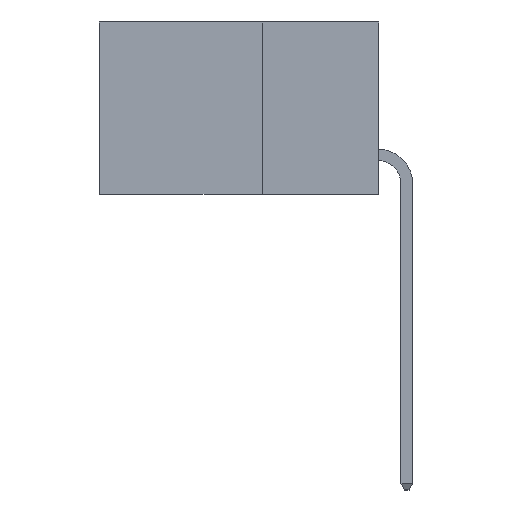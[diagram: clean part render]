
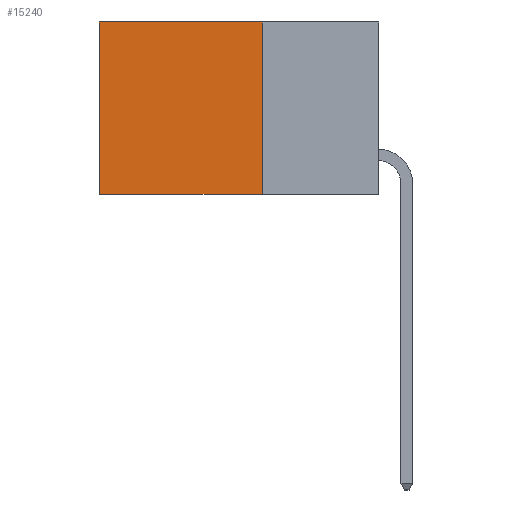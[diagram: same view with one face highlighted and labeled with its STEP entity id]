
A CAD part, left-side view. The second image highlights one B-rep face of the part: STEP entity #15240.
In plain terms, the highlighted planar face has unit normal (-1, 0, 0).
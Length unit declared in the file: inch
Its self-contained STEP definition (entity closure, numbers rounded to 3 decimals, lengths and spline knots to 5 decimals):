
#1170 = CARTESIAN_POINT ( 'NONE',  ( 0.2615, 0.6, -0.37 ) ) ;
#1968 = VERTEX_POINT ( 'NONE', #3800 ) ;
#2512 = LINE ( 'NONE', #5197, #6730 ) ;
#2752 = PLANE ( 'NONE',  #13616 ) ;
#3800 = CARTESIAN_POINT ( 'NONE',  ( 0.2615, 0.25, -0.37 ) ) ;
#5197 = CARTESIAN_POINT ( 'NONE',  ( 0.2615, 0.6, -0.37 ) ) ;
#5506 = VECTOR ( 'NONE', #15850, 39.37008 ) ;
#5813 = DIRECTION ( 'NONE',  ( 0., 0., -1. ) ) ;
#5832 = LINE ( 'NONE', #6506, #17611 ) ;
#6062 = VERTEX_POINT ( 'NONE', #12093 ) ;
#6355 = CARTESIAN_POINT ( 'NONE',  ( 0.2615, 0.25, -0.37 ) ) ;
#6506 = CARTESIAN_POINT ( 'NONE',  ( 0.2615, 0.25, 0. ) ) ;
#6730 = VECTOR ( 'NONE', #5813, 39.37008 ) ;
#7086 = EDGE_LOOP ( 'NONE', ( #19042, #13014, #13336, #17599 ) ) ;
#7244 = EDGE_CURVE ( 'NONE', #10485, #13763, #2512, .T. ) ;
#7478 = CARTESIAN_POINT ( 'NONE',  ( 0.2615, 0.25, -0.37 ) ) ;
#7992 = EDGE_CURVE ( 'NONE', #6062, #10485, #5832, .T. ) ;
#8607 = EDGE_CURVE ( 'NONE', #1968, #13763, #11613, .T. ) ;
#9054 = DIRECTION ( 'NONE',  ( 0., 0., -1. ) ) ;
#10485 = VERTEX_POINT ( 'NONE', #18209 ) ;
#11613 = LINE ( 'NONE', #6355, #14732 ) ;
#12093 = CARTESIAN_POINT ( 'NONE',  ( 0.2615, 0.25, 0. ) ) ;
#12482 = DIRECTION ( 'NONE',  ( 0., 1., 0. ) ) ;
#13014 = ORIENTED_EDGE ( 'NONE', *, *, #8607, .F. ) ;
#13336 = ORIENTED_EDGE ( 'NONE', *, *, #17713, .F. ) ;
#13616 = AXIS2_PLACEMENT_3D ( 'NONE', #7478, #18180, #9054 ) ;
#13763 = VERTEX_POINT ( 'NONE', #1170 ) ;
#14732 = VECTOR ( 'NONE', #12482, 39.37008 ) ;
#15240 = ADVANCED_FACE ( 'NONE', ( #16741 ), #2752, .F. ) ;
#15850 = DIRECTION ( 'NONE',  ( 0., 0., -1. ) ) ;
#16741 = FACE_OUTER_BOUND ( 'NONE', #7086, .T. ) ;
#17245 = DIRECTION ( 'NONE',  ( 0., 1., 0. ) ) ;
#17293 = CARTESIAN_POINT ( 'NONE',  ( 0.2615, 0.25, -0.37 ) ) ;
#17599 = ORIENTED_EDGE ( 'NONE', *, *, #7992, .T. ) ;
#17611 = VECTOR ( 'NONE', #17245, 39.37008 ) ;
#17713 = EDGE_CURVE ( 'NONE', #6062, #1968, #17770, .T. ) ;
#17770 = LINE ( 'NONE', #17293, #5506 ) ;
#18180 = DIRECTION ( 'NONE',  ( 1., 0., 0. ) ) ;
#18209 = CARTESIAN_POINT ( 'NONE',  ( 0.2615, 0.6, 0. ) ) ;
#19042 = ORIENTED_EDGE ( 'NONE', *, *, #7244, .T. ) ;
